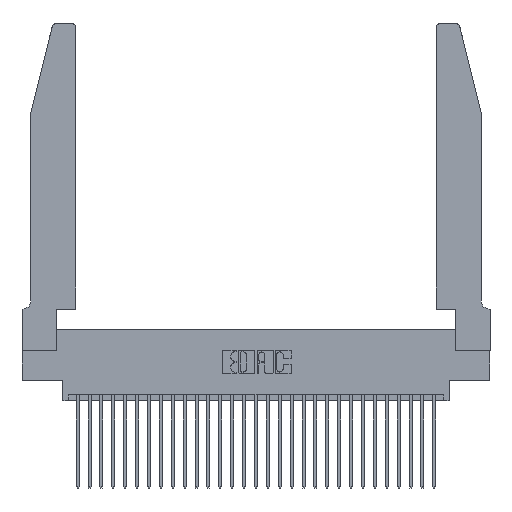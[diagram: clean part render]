
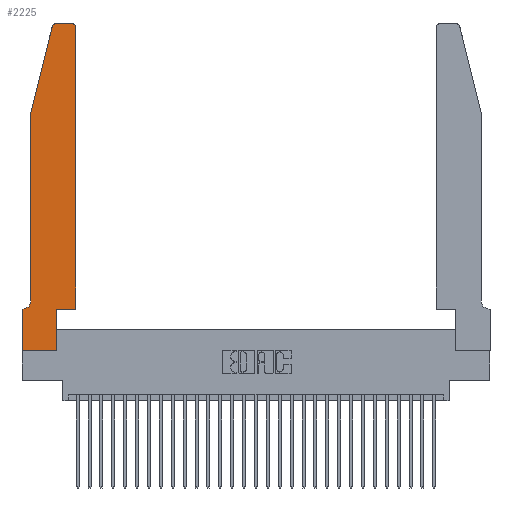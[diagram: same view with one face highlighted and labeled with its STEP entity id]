
A CAD part, top view. The second image highlights one B-rep face of the part: STEP entity #2225.
In plain terms, the highlighted planar face has unit normal (0, 0, 1).
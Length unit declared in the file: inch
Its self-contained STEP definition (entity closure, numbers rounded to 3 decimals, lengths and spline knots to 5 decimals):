
#961 = CARTESIAN_POINT ( 'NONE',  ( 0.4505, 2.72, 0.37 ) ) ;
#1418 = EDGE_CURVE ( 'NONE', #7467, #24608, #11495, .T. ) ;
#1620 = AXIS2_PLACEMENT_3D ( 'NONE', #12028, #9461, #23759 ) ;
#1917 = ORIENTED_EDGE ( 'NONE', *, *, #30492, .T. ) ;
#2225 = ADVANCED_FACE ( 'NONE', ( #22195 ), #2658, .T. ) ;
#2340 = VERTEX_POINT ( 'NONE', #15765 ) ;
#2516 = LINE ( 'NONE', #28810, #20358 ) ;
#2658 = PLANE ( 'NONE',  #13660 ) ;
#2846 = EDGE_CURVE ( 'NONE', #6521, #10801, #2516, .T. ) ;
#3476 = EDGE_CURVE ( 'NONE', #2340, #10054, #22481, .T. ) ;
#4653 = VECTOR ( 'NONE', #6324, 39.37008 ) ;
#4867 = DIRECTION ( 'NONE',  ( 0., 0., 1. ) ) ;
#5361 = DIRECTION ( 'NONE',  ( 0., -1., 0. ) ) ;
#6004 = DIRECTION ( 'NONE',  ( 0., 1., 0. ) ) ;
#6324 = DIRECTION ( 'NONE',  ( -1., 0., 0. ) ) ;
#6521 = VERTEX_POINT ( 'NONE', #18272 ) ;
#7159 = DIRECTION ( 'NONE',  ( 0., 0., 1. ) ) ;
#7467 = VERTEX_POINT ( 'NONE', #28095 ) ;
#8199 = DIRECTION ( 'NONE',  ( 0., 1., 0. ) ) ;
#8551 = AXIS2_PLACEMENT_3D ( 'NONE', #12029, #7159, #16604 ) ;
#9052 = EDGE_CURVE ( 'NONE', #22901, #17085, #25751, .T. ) ;
#9115 = EDGE_LOOP ( 'NONE', ( #9557, #21098, #24622, #11644, #23088, #19076, #1917, #15826, #24661, #22513, #27370, #15899 ) ) ;
#9132 = EDGE_CURVE ( 'NONE', #16342, #21619, #26452, .T. ) ;
#9461 = DIRECTION ( 'NONE',  ( 0., 0., -1. ) ) ;
#9516 = VECTOR ( 'NONE', #26806, 39.37008 ) ;
#9557 = ORIENTED_EDGE ( 'NONE', *, *, #9132, .T. ) ;
#9587 = EDGE_CURVE ( 'NONE', #21619, #6521, #29446, .T. ) ;
#10054 = VERTEX_POINT ( 'NONE', #19003 ) ;
#10131 = CARTESIAN_POINT ( 'NONE',  ( 0., 0., 0.37 ) ) ;
#10139 = VECTOR ( 'NONE', #13201, 39.37008 ) ;
#10186 = CARTESIAN_POINT ( 'NONE',  ( 0.0755, 2., 0.37 ) ) ;
#10759 = VECTOR ( 'NONE', #19198, 39.37008 ) ;
#10801 = VERTEX_POINT ( 'NONE', #15382 ) ;
#11421 = VERTEX_POINT ( 'NONE', #22916 ) ;
#11495 = LINE ( 'NONE', #21584, #10759 ) ;
#11644 = ORIENTED_EDGE ( 'NONE', *, *, #28089, .T. ) ;
#11696 = LINE ( 'NONE', #17239, #16569 ) ;
#11939 = DIRECTION ( 'NONE',  ( 1., 0., 0. ) ) ;
#12028 = CARTESIAN_POINT ( 'NONE',  ( 0.0055, 0.42, 0.37 ) ) ;
#12029 = CARTESIAN_POINT ( 'NONE',  ( 0.4205, 2.72, 0.37 ) ) ;
#12323 = DIRECTION ( 'NONE',  ( -0.239, -0.971, 0. ) ) ;
#12552 = CARTESIAN_POINT ( 'NONE',  ( 0., 0.35, 0.37 ) ) ;
#12661 = DIRECTION ( 'NONE',  ( 0., -1., 0. ) ) ;
#12716 = CARTESIAN_POINT ( 'NONE',  ( 0.284, 2.75, 0.37 ) ) ;
#12950 = AXIS2_PLACEMENT_3D ( 'NONE', #20301, #27623, #27819 ) ;
#13201 = DIRECTION ( 'NONE',  ( 1., 0., 0. ) ) ;
#13328 = CARTESIAN_POINT ( 'NONE',  ( 0.4505, 0.35, 0.37 ) ) ;
#13626 = CIRCLE ( 'NONE', #8551, 0.03 ) ;
#13660 = AXIS2_PLACEMENT_3D ( 'NONE', #16578, #4867, #11939 ) ;
#14011 = CARTESIAN_POINT ( 'NONE',  ( 0.4205, 2.75, 0.37 ) ) ;
#14108 = VECTOR ( 'NONE', #5361, 39.37008 ) ;
#14286 = VERTEX_POINT ( 'NONE', #17513 ) ;
#14959 = EDGE_CURVE ( 'NONE', #14286, #22901, #24257, .T. ) ;
#15293 = LINE ( 'NONE', #26703, #16786 ) ;
#15382 = CARTESIAN_POINT ( 'NONE',  ( 0.0755, 2., 0.37 ) ) ;
#15765 = CARTESIAN_POINT ( 'NONE',  ( 0., 0., 0.37 ) ) ;
#15826 = ORIENTED_EDGE ( 'NONE', *, *, #3476, .T. ) ;
#15899 = ORIENTED_EDGE ( 'NONE', *, *, #20177, .T. ) ;
#16342 = VERTEX_POINT ( 'NONE', #14011 ) ;
#16569 = VECTOR ( 'NONE', #12661, 39.37008 ) ;
#16578 = CARTESIAN_POINT ( 'NONE',  ( 0., 0.35, 0.37 ) ) ;
#16604 = DIRECTION ( 'NONE',  ( 1., 0., 0. ) ) ;
#16786 = VECTOR ( 'NONE', #8199, 39.37008 ) ;
#17085 = VERTEX_POINT ( 'NONE', #961 ) ;
#17239 = CARTESIAN_POINT ( 'NONE',  ( 0., 0., 0.37 ) ) ;
#17513 = CARTESIAN_POINT ( 'NONE',  ( 0.2865, 0.35, 0.37 ) ) ;
#17885 = CARTESIAN_POINT ( 'NONE',  ( 0.2605, 2.75, 0.37 ) ) ;
#18272 = CARTESIAN_POINT ( 'NONE',  ( 0.25487, 2.72718, 0.37 ) ) ;
#19003 = CARTESIAN_POINT ( 'NONE',  ( 0.2865, 0., 0.37 ) ) ;
#19076 = ORIENTED_EDGE ( 'NONE', *, *, #1418, .T. ) ;
#19198 = DIRECTION ( 'NONE',  ( -1., 0., 0. ) ) ;
#19446 = VECTOR ( 'NONE', #6004, 39.37008 ) ;
#20177 = EDGE_CURVE ( 'NONE', #17085, #16342, #13626, .T. ) ;
#20301 = CARTESIAN_POINT ( 'NONE',  ( 0.284, 2.72, 0.37 ) ) ;
#20358 = VECTOR ( 'NONE', #12323, 39.37008 ) ;
#21098 = ORIENTED_EDGE ( 'NONE', *, *, #9587, .T. ) ;
#21584 = CARTESIAN_POINT ( 'NONE',  ( 0.0755, 0.35, 0.37 ) ) ;
#21619 = VERTEX_POINT ( 'NONE', #12716 ) ;
#21768 = EDGE_CURVE ( 'NONE', #11421, #7467, #28661, .T. ) ;
#22182 = CARTESIAN_POINT ( 'NONE',  ( 0.4505, 0.35, 0.37 ) ) ;
#22195 = FACE_OUTER_BOUND ( 'NONE', #9115, .T. ) ;
#22209 = LINE ( 'NONE', #10186, #14108 ) ;
#22481 = LINE ( 'NONE', #10131, #9516 ) ;
#22513 = ORIENTED_EDGE ( 'NONE', *, *, #14959, .T. ) ;
#22901 = VERTEX_POINT ( 'NONE', #26364 ) ;
#22916 = CARTESIAN_POINT ( 'NONE',  ( 0.0755, 0.42, 0.37 ) ) ;
#23088 = ORIENTED_EDGE ( 'NONE', *, *, #21768, .T. ) ;
#23759 = DIRECTION ( 'NONE',  ( -1., 0., 0. ) ) ;
#24257 = LINE ( 'NONE', #22182, #10139 ) ;
#24608 = VERTEX_POINT ( 'NONE', #12552 ) ;
#24622 = ORIENTED_EDGE ( 'NONE', *, *, #2846, .T. ) ;
#24661 = ORIENTED_EDGE ( 'NONE', *, *, #27208, .T. ) ;
#25751 = LINE ( 'NONE', #13328, #19446 ) ;
#26364 = CARTESIAN_POINT ( 'NONE',  ( 0.4505, 0.35, 0.37 ) ) ;
#26452 = LINE ( 'NONE', #17885, #4653 ) ;
#26703 = CARTESIAN_POINT ( 'NONE',  ( 0.2865, 0.35, 0.37 ) ) ;
#26806 = DIRECTION ( 'NONE',  ( 1., 0., 0. ) ) ;
#27208 = EDGE_CURVE ( 'NONE', #10054, #14286, #15293, .T. ) ;
#27370 = ORIENTED_EDGE ( 'NONE', *, *, #9052, .T. ) ;
#27623 = DIRECTION ( 'NONE',  ( 0., 0., 1. ) ) ;
#27819 = DIRECTION ( 'NONE',  ( 1., 0., 0. ) ) ;
#28089 = EDGE_CURVE ( 'NONE', #10801, #11421, #22209, .T. ) ;
#28095 = CARTESIAN_POINT ( 'NONE',  ( 0.0055, 0.35, 0.37 ) ) ;
#28661 = CIRCLE ( 'NONE', #1620, 0.07 ) ;
#28810 = CARTESIAN_POINT ( 'NONE',  ( 0.0755, 2., 0.37 ) ) ;
#29446 = CIRCLE ( 'NONE', #12950, 0.03 ) ;
#30492 = EDGE_CURVE ( 'NONE', #24608, #2340, #11696, .T. ) ;
